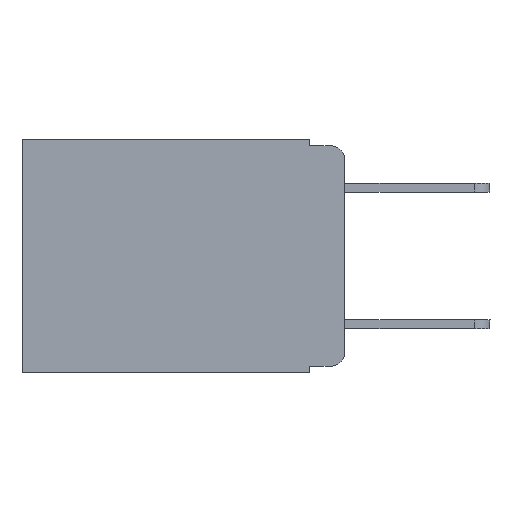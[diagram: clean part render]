
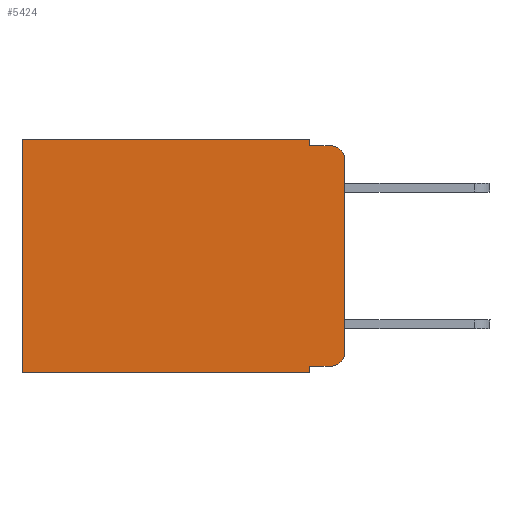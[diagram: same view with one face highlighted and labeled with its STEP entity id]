
A CAD part, left-side view. The second image highlights one B-rep face of the part: STEP entity #5424.
In plain terms, the highlighted planar face has unit normal (-1, 0, 0).
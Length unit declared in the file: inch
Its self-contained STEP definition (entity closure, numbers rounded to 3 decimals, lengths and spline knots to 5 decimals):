
#223 = CARTESIAN_POINT ( 'NONE',  ( 0.298, 0.02, -0.01 ) ) ;
#361 = VERTEX_POINT ( 'NONE', #14363 ) ;
#903 = CARTESIAN_POINT ( 'NONE',  ( 0.298, 0.051, -0.333 ) ) ;
#931 = DIRECTION ( 'NONE',  ( 0., 0., -1. ) ) ;
#1092 = CARTESIAN_POINT ( 'NONE',  ( 0.298, 0.051, -0.01 ) ) ;
#1220 = LINE ( 'NONE', #2429, #19799 ) ;
#1264 = ORIENTED_EDGE ( 'NONE', *, *, #11707, .T. ) ;
#1786 = CARTESIAN_POINT ( 'NONE',  ( 0.298, 0.473, 0. ) ) ;
#1906 = ORIENTED_EDGE ( 'NONE', *, *, #16864, .F. ) ;
#2106 = ORIENTED_EDGE ( 'NONE', *, *, #2408, .F. ) ;
#2366 = EDGE_CURVE ( 'NONE', #17783, #20446, #16443, .T. ) ;
#2395 = LINE ( 'NONE', #10935, #17593 ) ;
#2408 = EDGE_CURVE ( 'NONE', #2586, #12703, #10502, .T. ) ;
#2429 = CARTESIAN_POINT ( 'NONE',  ( 0.298, 0., 0. ) ) ;
#2586 = VERTEX_POINT ( 'NONE', #21572 ) ;
#2782 = LINE ( 'NONE', #1092, #22186 ) ;
#2811 = ORIENTED_EDGE ( 'NONE', *, *, #7066, .T. ) ;
#2910 = AXIS2_PLACEMENT_3D ( 'NONE', #19007, #7932, #931 ) ;
#3335 = CARTESIAN_POINT ( 'NONE',  ( 0.298, 0.473, -0.343 ) ) ;
#3725 = CARTESIAN_POINT ( 'NONE',  ( 0.298, 0., 0. ) ) ;
#3800 = DIRECTION ( 'NONE',  ( 0., 0., -1. ) ) ;
#3805 = VERTEX_POINT ( 'NONE', #16480 ) ;
#4243 = CARTESIAN_POINT ( 'NONE',  ( 0.298, 0.051, -0.01 ) ) ;
#4447 = CARTESIAN_POINT ( 'NONE',  ( 0.298, 0., -0.343 ) ) ;
#4467 = DIRECTION ( 'NONE',  ( 0., -1., 0. ) ) ;
#4722 = FACE_OUTER_BOUND ( 'NONE', #19857, .T. ) ;
#4967 = DIRECTION ( 'NONE',  ( -1., 0., 0. ) ) ;
#4975 = CARTESIAN_POINT ( 'NONE',  ( 0.298, 0.051, 0. ) ) ;
#5424 = ADVANCED_FACE ( 'NONE', ( #4722 ), #14847, .F. ) ;
#5528 = DIRECTION ( 'NONE',  ( 1., 0., 0. ) ) ;
#5537 = DIRECTION ( 'NONE',  ( 0., 1., 0. ) ) ;
#5961 = ORIENTED_EDGE ( 'NONE', *, *, #8418, .F. ) ;
#6004 = ORIENTED_EDGE ( 'NONE', *, *, #17033, .T. ) ;
#6110 = CARTESIAN_POINT ( 'NONE',  ( 0.298, 0., -0.03 ) ) ;
#6273 = DIRECTION ( 'NONE',  ( 0., 1., 0. ) ) ;
#6638 = AXIS2_PLACEMENT_3D ( 'NONE', #22733, #4967, #6851 ) ;
#6851 = DIRECTION ( 'NONE',  ( 0., 0., -1. ) ) ;
#7066 = EDGE_CURVE ( 'NONE', #21543, #12703, #9734, .T. ) ;
#7932 = DIRECTION ( 'NONE',  ( -1., 0., 0. ) ) ;
#8267 = ORIENTED_EDGE ( 'NONE', *, *, #19825, .F. ) ;
#8418 = EDGE_CURVE ( 'NONE', #18311, #9800, #2782, .T. ) ;
#8545 = LINE ( 'NONE', #4975, #16179 ) ;
#9433 = VERTEX_POINT ( 'NONE', #6110 ) ;
#9734 = LINE ( 'NONE', #1786, #22955 ) ;
#9800 = VERTEX_POINT ( 'NONE', #223 ) ;
#10502 = LINE ( 'NONE', #4447, #11644 ) ;
#10926 = DIRECTION ( 'NONE',  ( 0., 0., -1. ) ) ;
#10935 = CARTESIAN_POINT ( 'NONE',  ( 0.298, 0.051, 0. ) ) ;
#11644 = VECTOR ( 'NONE', #5537, 39.37008 ) ;
#11707 = EDGE_CURVE ( 'NONE', #3805, #21543, #1220, .T. ) ;
#12154 = DIRECTION ( 'NONE',  ( 0., 0., -1. ) ) ;
#12650 = DIRECTION ( 'NONE',  ( 0., -1., 0. ) ) ;
#12703 = VERTEX_POINT ( 'NONE', #3335 ) ;
#12857 = CARTESIAN_POINT ( 'NONE',  ( 0.298, 0.02, -0.333 ) ) ;
#12994 = VECTOR ( 'NONE', #19940, 39.37008 ) ;
#13097 = ORIENTED_EDGE ( 'NONE', *, *, #13156, .T. ) ;
#13156 = EDGE_CURVE ( 'NONE', #9433, #9800, #17762, .T. ) ;
#13189 = AXIS2_PLACEMENT_3D ( 'NONE', #3725, #5528, #3800 ) ;
#14363 = CARTESIAN_POINT ( 'NONE',  ( 0.298, 0., -0.313 ) ) ;
#14547 = CARTESIAN_POINT ( 'NONE',  ( 0.298, 0., 0. ) ) ;
#14828 = CIRCLE ( 'NONE', #2910, 0.02 ) ;
#14847 = PLANE ( 'NONE',  #13189 ) ;
#16179 = VECTOR ( 'NONE', #12154, 39.37008 ) ;
#16443 = LINE ( 'NONE', #21512, #23140 ) ;
#16480 = CARTESIAN_POINT ( 'NONE',  ( 0.298, 0.051, 0. ) ) ;
#16640 = LINE ( 'NONE', #14547, #12994 ) ;
#16864 = EDGE_CURVE ( 'NONE', #17783, #2586, #2395, .T. ) ;
#17033 = EDGE_CURVE ( 'NONE', #20446, #361, #14828, .T. ) ;
#17593 = VECTOR ( 'NONE', #18083, 39.37008 ) ;
#17762 = CIRCLE ( 'NONE', #6638, 0.02 ) ;
#17783 = VERTEX_POINT ( 'NONE', #903 ) ;
#17885 = EDGE_CURVE ( 'NONE', #3805, #18311, #8545, .T. ) ;
#18083 = DIRECTION ( 'NONE',  ( 0., 0., -1. ) ) ;
#18311 = VERTEX_POINT ( 'NONE', #4243 ) ;
#19007 = CARTESIAN_POINT ( 'NONE',  ( 0.298, 0.02, -0.313 ) ) ;
#19326 = CARTESIAN_POINT ( 'NONE',  ( 0.298, 0.473, 0. ) ) ;
#19799 = VECTOR ( 'NONE', #6273, 39.37008 ) ;
#19825 = EDGE_CURVE ( 'NONE', #9433, #361, #16640, .T. ) ;
#19857 = EDGE_LOOP ( 'NONE', ( #8267, #13097, #5961, #22844, #1264, #2811, #2106, #1906, #21990, #6004 ) ) ;
#19940 = DIRECTION ( 'NONE',  ( 0., 0., -1. ) ) ;
#20446 = VERTEX_POINT ( 'NONE', #12857 ) ;
#21512 = CARTESIAN_POINT ( 'NONE',  ( 0.298, 0.051, -0.333 ) ) ;
#21543 = VERTEX_POINT ( 'NONE', #19326 ) ;
#21572 = CARTESIAN_POINT ( 'NONE',  ( 0.298, 0.051, -0.343 ) ) ;
#21990 = ORIENTED_EDGE ( 'NONE', *, *, #2366, .T. ) ;
#22186 = VECTOR ( 'NONE', #4467, 39.37008 ) ;
#22733 = CARTESIAN_POINT ( 'NONE',  ( 0.298, 0.02, -0.03 ) ) ;
#22844 = ORIENTED_EDGE ( 'NONE', *, *, #17885, .F. ) ;
#22955 = VECTOR ( 'NONE', #10926, 39.37008 ) ;
#23140 = VECTOR ( 'NONE', #12650, 39.37008 ) ;
